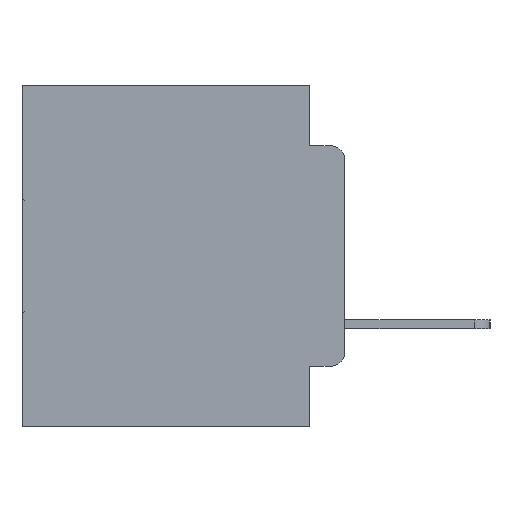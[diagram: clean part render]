
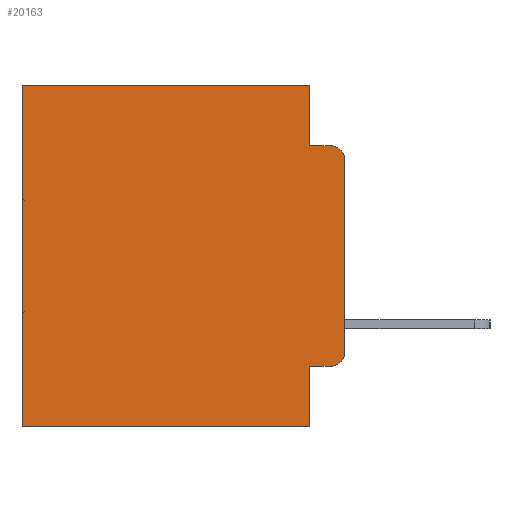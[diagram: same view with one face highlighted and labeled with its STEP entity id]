
A CAD part, left-side view. The second image highlights one B-rep face of the part: STEP entity #20163.
In plain terms, the highlighted planar face has unit normal (-1, 0, 0).
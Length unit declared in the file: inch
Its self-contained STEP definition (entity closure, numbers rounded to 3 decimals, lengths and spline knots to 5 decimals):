
#789 = ORIENTED_EDGE ( 'NONE', *, *, #3448, .F. ) ;
#963 = VERTEX_POINT ( 'NONE', #12601 ) ;
#971 = LINE ( 'NONE', #28024, #6794 ) ;
#1906 = VECTOR ( 'NONE', #5484, 39.37008 ) ;
#2280 = LINE ( 'NONE', #2814, #14733 ) ;
#2633 = CARTESIAN_POINT ( 'NONE',  ( 0.298, 0.02, -0.1085 ) ) ;
#2814 = CARTESIAN_POINT ( 'NONE',  ( 0.298, 0.051, 0. ) ) ;
#2984 = VERTEX_POINT ( 'NONE', #15834 ) ;
#3448 = EDGE_CURVE ( 'NONE', #963, #11073, #18863, .T. ) ;
#3564 = CIRCLE ( 'NONE', #29629, 0.02 ) ;
#5122 = DIRECTION ( 'NONE',  ( 0., 0., -1. ) ) ;
#5269 = CARTESIAN_POINT ( 'NONE',  ( 0.298, 0.051, -0.0885 ) ) ;
#5380 = DIRECTION ( 'NONE',  ( 0., -1., 0. ) ) ;
#5484 = DIRECTION ( 'NONE',  ( 0., -1., 0. ) ) ;
#5845 = VERTEX_POINT ( 'NONE', #19201 ) ;
#5953 = EDGE_LOOP ( 'NONE', ( #19665, #20250, #789, #25227, #7176, #29307, #10589, #9359, #30948, #8035 ) ) ;
#6794 = VECTOR ( 'NONE', #10880, 39.37008 ) ;
#6865 = CIRCLE ( 'NONE', #18790, 0.02 ) ;
#7176 = ORIENTED_EDGE ( 'NONE', *, *, #28700, .T. ) ;
#8035 = ORIENTED_EDGE ( 'NONE', *, *, #28161, .T. ) ;
#8399 = EDGE_CURVE ( 'NONE', #5845, #963, #971, .T. ) ;
#8849 = DIRECTION ( 'NONE',  ( 0., 0., -1. ) ) ;
#9343 = VECTOR ( 'NONE', #8849, 39.37008 ) ;
#9359 = ORIENTED_EDGE ( 'NONE', *, *, #21679, .F. ) ;
#9543 = VERTEX_POINT ( 'NONE', #20449 ) ;
#10292 = DIRECTION ( 'NONE',  ( 0., 0., -1. ) ) ;
#10589 = ORIENTED_EDGE ( 'NONE', *, *, #24103, .F. ) ;
#10795 = CARTESIAN_POINT ( 'NONE',  ( 0.298, 0.02, -0.3915 ) ) ;
#10880 = DIRECTION ( 'NONE',  ( 0., 0., -1. ) ) ;
#10999 = DIRECTION ( 'NONE',  ( 0., 0., -1. ) ) ;
#11073 = VERTEX_POINT ( 'NONE', #14216 ) ;
#12058 = LINE ( 'NONE', #17838, #24366 ) ;
#12252 = VECTOR ( 'NONE', #5380, 39.37008 ) ;
#12601 = CARTESIAN_POINT ( 'NONE',  ( 0.298, 0.051, -0.0885 ) ) ;
#13290 = DIRECTION ( 'NONE',  ( 0., 0., -1. ) ) ;
#13864 = PLANE ( 'NONE',  #27605 ) ;
#14216 = CARTESIAN_POINT ( 'NONE',  ( 0.298, 0.02, -0.0885 ) ) ;
#14669 = VERTEX_POINT ( 'NONE', #22078 ) ;
#14733 = VECTOR ( 'NONE', #10292, 39.37008 ) ;
#15092 = EDGE_CURVE ( 'NONE', #14669, #19644, #15966, .T. ) ;
#15333 = DIRECTION ( 'NONE',  ( 0., 1., 0. ) ) ;
#15834 = CARTESIAN_POINT ( 'NONE',  ( 0.298, 0., -0.1085 ) ) ;
#15966 = LINE ( 'NONE', #16263, #9343 ) ;
#16263 = CARTESIAN_POINT ( 'NONE',  ( 0.298, 0.473, 0. ) ) ;
#16328 = CARTESIAN_POINT ( 'NONE',  ( 0.298, 0., -0.3915 ) ) ;
#16357 = DIRECTION ( 'NONE',  ( 0., 0., -1. ) ) ;
#16748 = EDGE_CURVE ( 'NONE', #9543, #17258, #20914, .T. ) ;
#17258 = VERTEX_POINT ( 'NONE', #31682 ) ;
#17838 = CARTESIAN_POINT ( 'NONE',  ( 0.298, 0., 0. ) ) ;
#18790 = AXIS2_PLACEMENT_3D ( 'NONE', #2633, #19977, #5122 ) ;
#18863 = LINE ( 'NONE', #5269, #12252 ) ;
#18867 = VECTOR ( 'NONE', #24649, 39.37008 ) ;
#19108 = CARTESIAN_POINT ( 'NONE',  ( 0.298, 0.473, -0.5 ) ) ;
#19201 = CARTESIAN_POINT ( 'NONE',  ( 0.298, 0.051, 0. ) ) ;
#19644 = VERTEX_POINT ( 'NONE', #19108 ) ;
#19665 = ORIENTED_EDGE ( 'NONE', *, *, #27163, .F. ) ;
#19953 = VERTEX_POINT ( 'NONE', #22822 ) ;
#19977 = DIRECTION ( 'NONE',  ( -1., 0., 0. ) ) ;
#20163 = ADVANCED_FACE ( 'NONE', ( #27440 ), #13864, .F. ) ;
#20250 = ORIENTED_EDGE ( 'NONE', *, *, #30319, .T. ) ;
#20449 = CARTESIAN_POINT ( 'NONE',  ( 0.298, 0.051, -0.4115 ) ) ;
#20914 = LINE ( 'NONE', #25784, #1906 ) ;
#21679 = EDGE_CURVE ( 'NONE', #9543, #19953, #2280, .T. ) ;
#21771 = VECTOR ( 'NONE', #10999, 39.37008 ) ;
#22078 = CARTESIAN_POINT ( 'NONE',  ( 0.298, 0.473, 0. ) ) ;
#22214 = CARTESIAN_POINT ( 'NONE',  ( 0.298, 0., -0.5 ) ) ;
#22822 = CARTESIAN_POINT ( 'NONE',  ( 0.298, 0.051, -0.5 ) ) ;
#23277 = CARTESIAN_POINT ( 'NONE',  ( 0.298, 0., 0. ) ) ;
#24103 = EDGE_CURVE ( 'NONE', #19953, #19644, #31644, .T. ) ;
#24366 = VECTOR ( 'NONE', #15333, 39.37008 ) ;
#24649 = DIRECTION ( 'NONE',  ( 0., 1., 0. ) ) ;
#25227 = ORIENTED_EDGE ( 'NONE', *, *, #8399, .F. ) ;
#25784 = CARTESIAN_POINT ( 'NONE',  ( 0.298, 0.051, -0.4115 ) ) ;
#27163 = EDGE_CURVE ( 'NONE', #2984, #28289, #28198, .T. ) ;
#27440 = FACE_OUTER_BOUND ( 'NONE', #5953, .T. ) ;
#27605 = AXIS2_PLACEMENT_3D ( 'NONE', #28483, #30835, #16357 ) ;
#27944 = DIRECTION ( 'NONE',  ( -1., 0., 0. ) ) ;
#28024 = CARTESIAN_POINT ( 'NONE',  ( 0.298, 0.051, 0. ) ) ;
#28161 = EDGE_CURVE ( 'NONE', #17258, #28289, #3564, .T. ) ;
#28198 = LINE ( 'NONE', #23277, #21771 ) ;
#28289 = VERTEX_POINT ( 'NONE', #16328 ) ;
#28483 = CARTESIAN_POINT ( 'NONE',  ( 0.298, 0., 0. ) ) ;
#28700 = EDGE_CURVE ( 'NONE', #5845, #14669, #12058, .T. ) ;
#29307 = ORIENTED_EDGE ( 'NONE', *, *, #15092, .T. ) ;
#29629 = AXIS2_PLACEMENT_3D ( 'NONE', #10795, #27944, #13290 ) ;
#30319 = EDGE_CURVE ( 'NONE', #2984, #11073, #6865, .T. ) ;
#30835 = DIRECTION ( 'NONE',  ( 1., 0., 0. ) ) ;
#30948 = ORIENTED_EDGE ( 'NONE', *, *, #16748, .T. ) ;
#31644 = LINE ( 'NONE', #22214, #18867 ) ;
#31682 = CARTESIAN_POINT ( 'NONE',  ( 0.298, 0.02, -0.4115 ) ) ;
